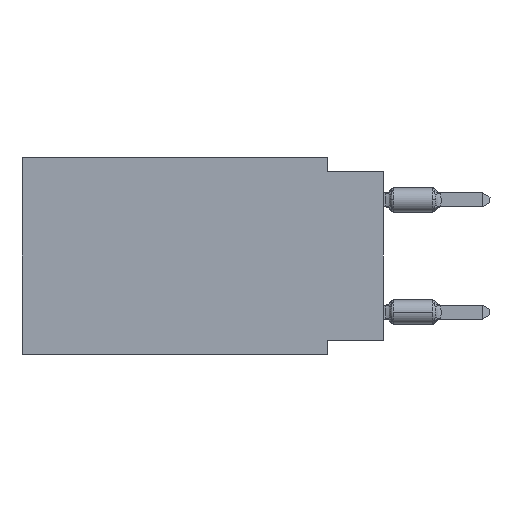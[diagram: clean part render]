
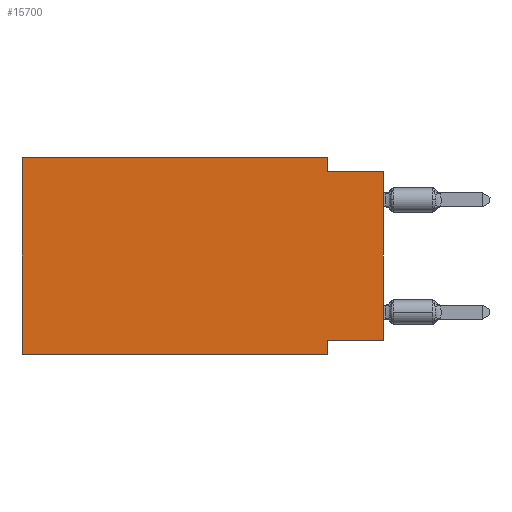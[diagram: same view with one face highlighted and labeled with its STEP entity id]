
A CAD part, left-side view. The second image highlights one B-rep face of the part: STEP entity #15700.
In plain terms, the highlighted planar face has unit normal (-1, 0, 0).
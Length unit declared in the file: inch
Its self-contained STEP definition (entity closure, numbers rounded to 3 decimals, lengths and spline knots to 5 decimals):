
#767 = CARTESIAN_POINT ( 'NONE',  ( 0., 0.1, -0.325 ) ) ;
#797 = ORIENTED_EDGE ( 'NONE', *, *, #2550, .F. ) ;
#910 = CARTESIAN_POINT ( 'NONE',  ( 0., 0.1, -0.025 ) ) ;
#2147 = VERTEX_POINT ( 'NONE', #10927 ) ;
#2519 = EDGE_CURVE ( 'NONE', #7162, #12651, #9767, .T. ) ;
#2550 = EDGE_CURVE ( 'NONE', #13535, #11949, #4604, .T. ) ;
#2698 = EDGE_CURVE ( 'NONE', #9007, #15393, #5095, .T. ) ;
#2699 = LINE ( 'NONE', #9144, #9653 ) ;
#3119 = DIRECTION ( 'NONE',  ( 0., -1., 0. ) ) ;
#3197 = CARTESIAN_POINT ( 'NONE',  ( 0., 0.1, -0.35 ) ) ;
#3742 = DIRECTION ( 'NONE',  ( 0., -1., 0. ) ) ;
#3800 = CARTESIAN_POINT ( 'NONE',  ( 0., 0.1, 0. ) ) ;
#4382 = CARTESIAN_POINT ( 'NONE',  ( 0., 0.645, -0.35 ) ) ;
#4443 = DIRECTION ( 'NONE',  ( 0., 0., -1. ) ) ;
#4572 = LINE ( 'NONE', #8216, #4588 ) ;
#4588 = VECTOR ( 'NONE', #9823, 39.37008 ) ;
#4604 = LINE ( 'NONE', #8501, #11308 ) ;
#4709 = ORIENTED_EDGE ( 'NONE', *, *, #11948, .T. ) ;
#5010 = CARTESIAN_POINT ( 'NONE',  ( 0., 0.645, 0. ) ) ;
#5095 = LINE ( 'NONE', #5010, #6146 ) ;
#5235 = DIRECTION ( 'NONE',  ( 0., 0., 1. ) ) ;
#5521 = PLANE ( 'NONE',  #14064 ) ;
#5644 = LINE ( 'NONE', #4382, #14945 ) ;
#6146 = VECTOR ( 'NONE', #3742, 39.37008 ) ;
#7162 = VERTEX_POINT ( 'NONE', #910 ) ;
#7975 = DIRECTION ( 'NONE',  ( 1., 0., 0. ) ) ;
#8216 = CARTESIAN_POINT ( 'NONE',  ( 0., 0., 0. ) ) ;
#8247 = DIRECTION ( 'NONE',  ( 0., -1., 0. ) ) ;
#8501 = CARTESIAN_POINT ( 'NONE',  ( 0., 0.1, -0.35 ) ) ;
#8970 = DIRECTION ( 'NONE',  ( 0., 0., -1. ) ) ;
#9007 = VERTEX_POINT ( 'NONE', #14985 ) ;
#9144 = CARTESIAN_POINT ( 'NONE',  ( 0., 0.645, 0. ) ) ;
#9187 = ORIENTED_EDGE ( 'NONE', *, *, #10382, .F. ) ;
#9233 = ORIENTED_EDGE ( 'NONE', *, *, #16639, .F. ) ;
#9448 = CARTESIAN_POINT ( 'NONE',  ( 0., 0.1, 0. ) ) ;
#9482 = VECTOR ( 'NONE', #8970, 39.37008 ) ;
#9653 = VECTOR ( 'NONE', #5235, 39.37008 ) ;
#9690 = CARTESIAN_POINT ( 'NONE',  ( 0., 0., -0.025 ) ) ;
#9767 = LINE ( 'NONE', #9690, #15671 ) ;
#9823 = DIRECTION ( 'NONE',  ( 0., 0., 1. ) ) ;
#10274 = CARTESIAN_POINT ( 'NONE',  ( 0., 0., -0.325 ) ) ;
#10382 = EDGE_CURVE ( 'NONE', #12668, #9007, #2699, .T. ) ;
#10443 = CARTESIAN_POINT ( 'NONE',  ( 0., 0.645, 0. ) ) ;
#10699 = DIRECTION ( 'NONE',  ( 0., 0., -1. ) ) ;
#10927 = CARTESIAN_POINT ( 'NONE',  ( 0., 0., -0.325 ) ) ;
#11308 = VECTOR ( 'NONE', #4443, 39.37008 ) ;
#11470 = LINE ( 'NONE', #10274, #11622 ) ;
#11622 = VECTOR ( 'NONE', #12578, 39.37008 ) ;
#11636 = CARTESIAN_POINT ( 'NONE',  ( 0., 0., -0.025 ) ) ;
#11948 = EDGE_CURVE ( 'NONE', #12668, #11949, #5644, .T. ) ;
#11949 = VERTEX_POINT ( 'NONE', #3197 ) ;
#12578 = DIRECTION ( 'NONE',  ( 0., 1., 0. ) ) ;
#12651 = VERTEX_POINT ( 'NONE', #11636 ) ;
#12668 = VERTEX_POINT ( 'NONE', #14278 ) ;
#12944 = ORIENTED_EDGE ( 'NONE', *, *, #16236, .T. ) ;
#12963 = LINE ( 'NONE', #3800, #9482 ) ;
#13535 = VERTEX_POINT ( 'NONE', #767 ) ;
#14032 = ORIENTED_EDGE ( 'NONE', *, *, #2519, .F. ) ;
#14064 = AXIS2_PLACEMENT_3D ( 'NONE', #10443, #7975, #10699 ) ;
#14094 = ORIENTED_EDGE ( 'NONE', *, *, #2698, .F. ) ;
#14278 = CARTESIAN_POINT ( 'NONE',  ( 0., 0.645, -0.35 ) ) ;
#14945 = VECTOR ( 'NONE', #3119, 39.37008 ) ;
#14985 = CARTESIAN_POINT ( 'NONE',  ( 0., 0.645, 0. ) ) ;
#15393 = VERTEX_POINT ( 'NONE', #9448 ) ;
#15591 = EDGE_CURVE ( 'NONE', #2147, #13535, #11470, .T. ) ;
#15671 = VECTOR ( 'NONE', #8247, 39.37008 ) ;
#15700 = ADVANCED_FACE ( 'NONE', ( #15887 ), #5521, .F. ) ;
#15794 = EDGE_LOOP ( 'NONE', ( #12944, #14032, #9233, #14094, #9187, #4709, #797, #16350 ) ) ;
#15887 = FACE_OUTER_BOUND ( 'NONE', #15794, .T. ) ;
#16236 = EDGE_CURVE ( 'NONE', #2147, #12651, #4572, .T. ) ;
#16350 = ORIENTED_EDGE ( 'NONE', *, *, #15591, .F. ) ;
#16639 = EDGE_CURVE ( 'NONE', #15393, #7162, #12963, .T. ) ;
